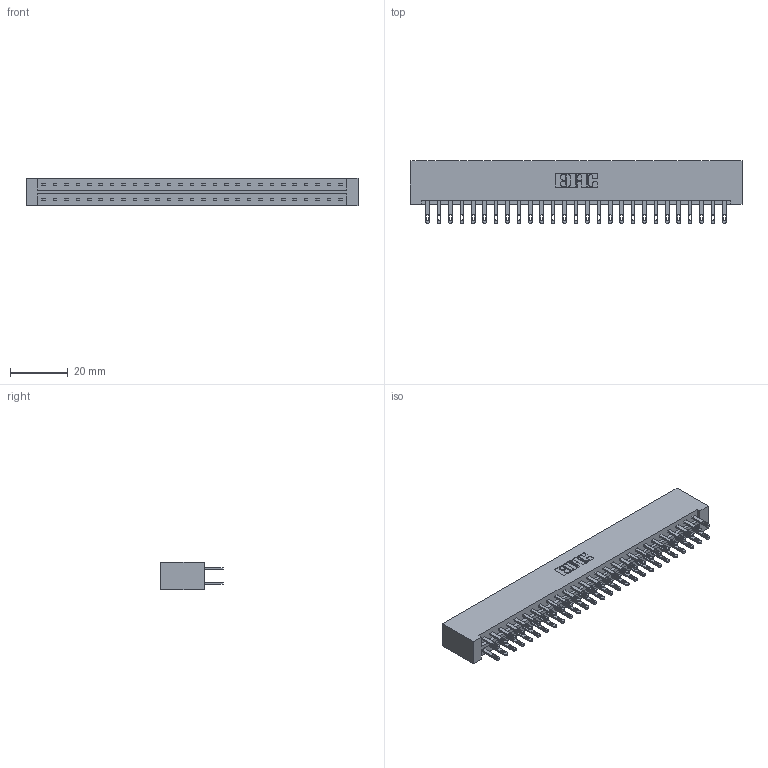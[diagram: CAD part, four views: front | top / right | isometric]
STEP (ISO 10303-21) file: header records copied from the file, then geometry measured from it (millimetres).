
FILE_DESCRIPTION (( 'STEP AP203' ), '1' );
FILE_NAME ('833-054-500-201.STEP', '2020-06-04T20:13:49', ( '' ), ( '' ), 'SwSTEP 2.0', 'SolidWorks 2020', '' );
FILE_SCHEMA (( 'CONFIG_CONTROL_DESIGN' ));
Length unit declared in the file: inch
Products named in the file (3): 345-292-001_345-293-100; 833-054-500-201; 833 Part_Lugless
Assembly tree (55 placements, depth 2):
  833-054-500-201
    833 Part_Lugless
    345-292-001_345-293-100  x54
Bounding box: 115.24 x 21.85 x 9.4 mm (x, y, z)
Volume: 12422.3 mm3; surface area: 15143.7 mm2
Topology: 55 solids, 55 shells, 2698 faces, 8225 edges, 5482 vertices
Faces by surface type: plane 1686, cylinder 1012
Entity records: 18963 total; most frequent: CARTESIAN_POINT 3158, ORIENTED_EDGE 3094, DIRECTION 2719, EDGE_CURVE 1547, LINE 1423, VECTOR 1423, VERTEX_POINT 1030, AXIS2_PLACEMENT_3D 648
